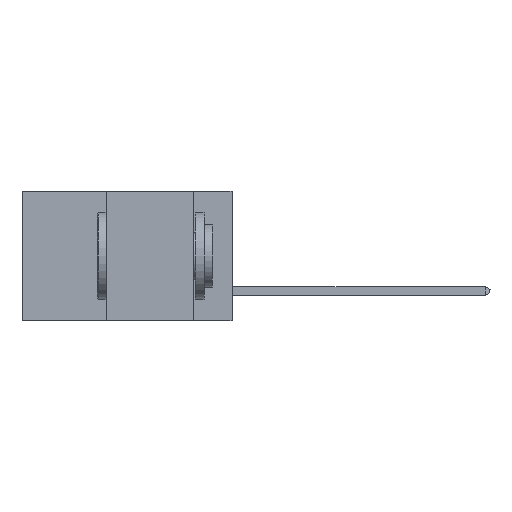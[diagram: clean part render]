
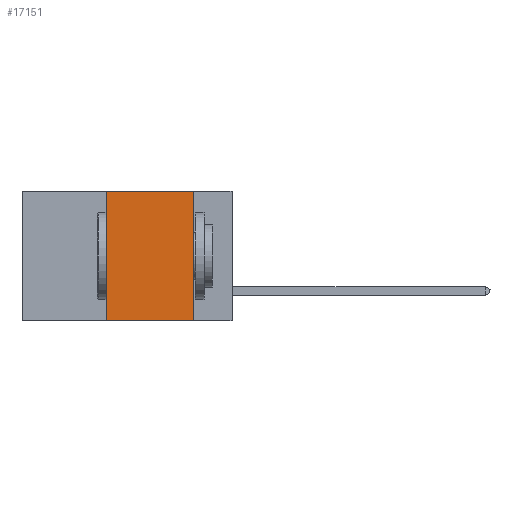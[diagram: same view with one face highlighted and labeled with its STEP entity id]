
A CAD part, left-side view. The second image highlights one B-rep face of the part: STEP entity #17151.
In plain terms, the highlighted planar face has unit normal (-1, 0, 0).
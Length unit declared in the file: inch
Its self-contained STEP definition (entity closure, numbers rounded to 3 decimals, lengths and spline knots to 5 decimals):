
#35 = VERTEX_POINT ( 'NONE', #23531 ) ;
#56 = LINE ( 'NONE', #6931, #20280 ) ;
#596 = CARTESIAN_POINT ( 'NONE',  ( 0., 0.6, 0. ) ) ;
#860 = EDGE_CURVE ( 'NONE', #17629, #26605, #22502, .T. ) ;
#1670 = LINE ( 'NONE', #4713, #23583 ) ;
#1746 = VERTEX_POINT ( 'NONE', #2720 ) ;
#1846 = VECTOR ( 'NONE', #23854, 39.37008 ) ;
#2359 = DIRECTION ( 'NONE',  ( 0., 0., 1. ) ) ;
#2661 = CARTESIAN_POINT ( 'NONE',  ( 0., 0.6, 0. ) ) ;
#2720 = CARTESIAN_POINT ( 'NONE',  ( 0., 0.36, 0. ) ) ;
#4713 = CARTESIAN_POINT ( 'NONE',  ( 0., 0.6, -0.37 ) ) ;
#6779 = DIRECTION ( 'NONE',  ( 0., -1., 0. ) ) ;
#6931 = CARTESIAN_POINT ( 'NONE',  ( 0., 0.36, 0. ) ) ;
#9861 = ORIENTED_EDGE ( 'NONE', *, *, #11622, .T. ) ;
#9956 = CARTESIAN_POINT ( 'NONE',  ( 0., 0.11, 0. ) ) ;
#11072 = DIRECTION ( 'NONE',  ( 0., 0., -1. ) ) ;
#11622 = EDGE_CURVE ( 'NONE', #35, #26605, #1670, .T. ) ;
#11810 = CARTESIAN_POINT ( 'NONE',  ( 0., 0.11, 0. ) ) ;
#13234 = PLANE ( 'NONE',  #17616 ) ;
#15922 = EDGE_CURVE ( 'NONE', #35, #1746, #56, .T. ) ;
#17151 = ADVANCED_FACE ( 'NONE', ( #26858 ), #13234, .F. ) ;
#17410 = ORIENTED_EDGE ( 'NONE', *, *, #860, .F. ) ;
#17616 = AXIS2_PLACEMENT_3D ( 'NONE', #2661, #23838, #11072 ) ;
#17629 = VERTEX_POINT ( 'NONE', #11810 ) ;
#17766 = LINE ( 'NONE', #596, #1846 ) ;
#17860 = CARTESIAN_POINT ( 'NONE',  ( 0., 0.11, -0.37 ) ) ;
#20280 = VECTOR ( 'NONE', #2359, 39.37008 ) ;
#21521 = EDGE_LOOP ( 'NONE', ( #17410, #27687, #26276, #9861 ) ) ;
#22449 = EDGE_CURVE ( 'NONE', #1746, #17629, #17766, .T. ) ;
#22502 = LINE ( 'NONE', #9956, #24817 ) ;
#23531 = CARTESIAN_POINT ( 'NONE',  ( 0., 0.36, -0.37 ) ) ;
#23583 = VECTOR ( 'NONE', #6779, 39.37008 ) ;
#23838 = DIRECTION ( 'NONE',  ( 1., 0., 0. ) ) ;
#23854 = DIRECTION ( 'NONE',  ( 0., -1., 0. ) ) ;
#24817 = VECTOR ( 'NONE', #25013, 39.37008 ) ;
#25013 = DIRECTION ( 'NONE',  ( 0., 0., -1. ) ) ;
#26276 = ORIENTED_EDGE ( 'NONE', *, *, #15922, .F. ) ;
#26605 = VERTEX_POINT ( 'NONE', #17860 ) ;
#26858 = FACE_OUTER_BOUND ( 'NONE', #21521, .T. ) ;
#27687 = ORIENTED_EDGE ( 'NONE', *, *, #22449, .F. ) ;
